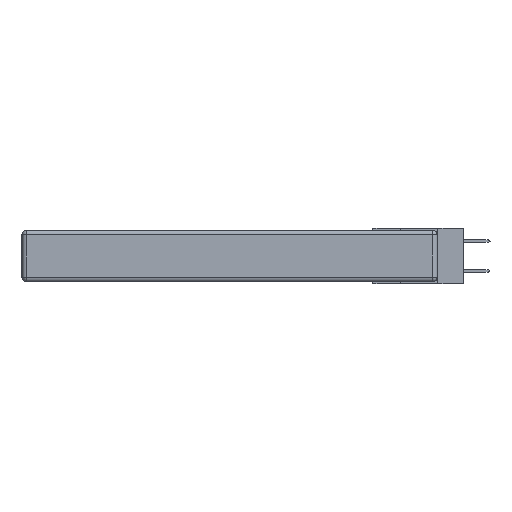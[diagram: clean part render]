
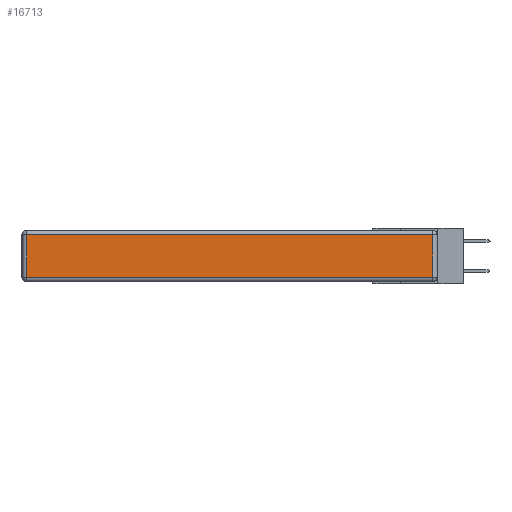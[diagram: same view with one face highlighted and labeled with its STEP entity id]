
A CAD part, left-side view. The second image highlights one B-rep face of the part: STEP entity #16713.
In plain terms, the highlighted planar face has unit normal (-1, 0, 0).
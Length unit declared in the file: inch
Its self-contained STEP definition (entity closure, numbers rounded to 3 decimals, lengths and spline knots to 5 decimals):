
#201 = EDGE_LOOP ( 'NONE', ( #10421, #17743, #12519, #17611 ) ) ;
#489 = LINE ( 'NONE', #16158, #8887 ) ;
#2535 = CARTESIAN_POINT ( 'NONE',  ( 0., 2.72, -0.03 ) ) ;
#2634 = CARTESIAN_POINT ( 'NONE',  ( 0., 2.75, -0.03 ) ) ;
#3538 = CARTESIAN_POINT ( 'NONE',  ( 0., 0.03, -0.313 ) ) ;
#4172 = VERTEX_POINT ( 'NONE', #3538 ) ;
#4748 = VECTOR ( 'NONE', #8876, 39.37008 ) ;
#5681 = DIRECTION ( 'NONE',  ( -1., 0., 0. ) ) ;
#5857 = LINE ( 'NONE', #16181, #4748 ) ;
#6986 = PLANE ( 'NONE',  #7045 ) ;
#7045 = AXIS2_PLACEMENT_3D ( 'NONE', #11313, #5681, #8672 ) ;
#8222 = DIRECTION ( 'NONE',  ( 0., 1., 0. ) ) ;
#8672 = DIRECTION ( 'NONE',  ( 0., 0., 1. ) ) ;
#8787 = DIRECTION ( 'NONE',  ( 0., 0., 1. ) ) ;
#8876 = DIRECTION ( 'NONE',  ( 0., 0., -1. ) ) ;
#8887 = VECTOR ( 'NONE', #8787, 39.37008 ) ;
#10050 = LINE ( 'NONE', #12392, #17985 ) ;
#10421 = ORIENTED_EDGE ( 'NONE', *, *, #15406, .T. ) ;
#11261 = DIRECTION ( 'NONE',  ( 0., -1., 0. ) ) ;
#11313 = CARTESIAN_POINT ( 'NONE',  ( 0., 0., -0.343 ) ) ;
#12392 = CARTESIAN_POINT ( 'NONE',  ( 0., 0., -0.313 ) ) ;
#12519 = ORIENTED_EDGE ( 'NONE', *, *, #15487, .T. ) ;
#12960 = VECTOR ( 'NONE', #8222, 39.37008 ) ;
#13669 = EDGE_CURVE ( 'NONE', #4172, #13706, #489, .T. ) ;
#13706 = VERTEX_POINT ( 'NONE', #16417 ) ;
#13764 = CARTESIAN_POINT ( 'NONE',  ( 0., 2.72, -0.313 ) ) ;
#15406 = EDGE_CURVE ( 'NONE', #15970, #4172, #10050, .T. ) ;
#15487 = EDGE_CURVE ( 'NONE', #13706, #16359, #18663, .T. ) ;
#15970 = VERTEX_POINT ( 'NONE', #13764 ) ;
#16158 = CARTESIAN_POINT ( 'NONE',  ( 0., 0.03, -0.343 ) ) ;
#16181 = CARTESIAN_POINT ( 'NONE',  ( 0., 2.72, -0.343 ) ) ;
#16359 = VERTEX_POINT ( 'NONE', #2535 ) ;
#16417 = CARTESIAN_POINT ( 'NONE',  ( 0., 0.03, -0.03 ) ) ;
#16713 = ADVANCED_FACE ( 'NONE', ( #17952 ), #6986, .T. ) ;
#17611 = ORIENTED_EDGE ( 'NONE', *, *, #18400, .T. ) ;
#17743 = ORIENTED_EDGE ( 'NONE', *, *, #13669, .T. ) ;
#17952 = FACE_OUTER_BOUND ( 'NONE', #201, .T. ) ;
#17985 = VECTOR ( 'NONE', #11261, 39.37008 ) ;
#18400 = EDGE_CURVE ( 'NONE', #16359, #15970, #5857, .T. ) ;
#18663 = LINE ( 'NONE', #2634, #12960 ) ;
